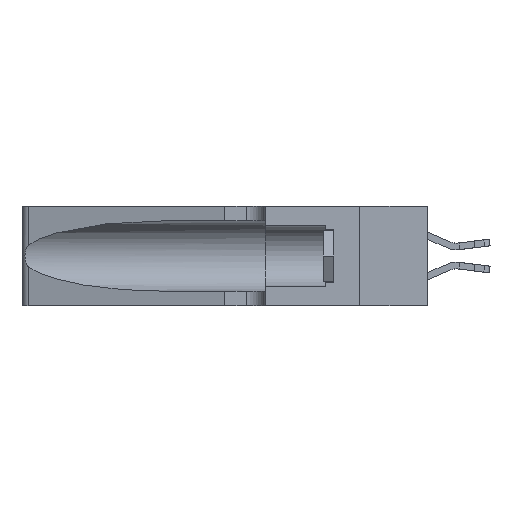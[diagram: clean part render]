
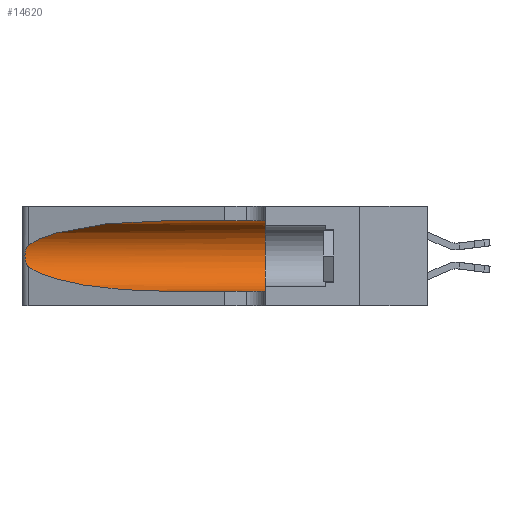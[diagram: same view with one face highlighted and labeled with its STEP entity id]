
A CAD part, left-side view. The second image highlights one B-rep face of the part: STEP entity #14620.
In plain terms, the highlighted cylindrical face has radius 3.308 mm (diameter 6.617 mm), a partial arc.
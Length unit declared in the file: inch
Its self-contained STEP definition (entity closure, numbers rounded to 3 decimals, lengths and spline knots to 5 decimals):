
#115 = LINE ( 'NONE', #6173, #20136 ) ;
#243 =( BOUNDED_CURVE ( )  B_SPLINE_CURVE ( 3, ( #4963, #20373, #3072, #16593 ),
 .UNSPECIFIED., .F., .F. ) 
 B_SPLINE_CURVE_WITH_KNOTS ( ( 4, 4 ),
 ( 3.44316, 4.71239 ),
 .UNSPECIFIED. ) 
 CURVE ( )  GEOMETRIC_REPRESENTATION_ITEM ( )  RATIONAL_B_SPLINE_CURVE ( ( 1., 0.87, 0.87, 1. ) ) 
 REPRESENTATION_ITEM ( '' )  );
#490 = ORIENTED_EDGE ( 'NONE', *, *, #7059, .T. ) ;
#665 = DIRECTION ( 'NONE',  ( 0., 0., -1. ) ) ;
#740 = VERTEX_POINT ( 'NONE', #21067 ) ;
#1482 = CARTESIAN_POINT ( 'NONE',  ( 0.25639, 1.23186, 0.15144 ) ) ;
#2315 =( BOUNDED_CURVE ( )  B_SPLINE_CURVE ( 3, ( #17032, #24825, #15292, #3704 ),
 .UNSPECIFIED., .F., .F. ) 
 B_SPLINE_CURVE_WITH_KNOTS ( ( 4, 4 ),
 ( 1.5708, 2.84003 ),
 .UNSPECIFIED. ) 
 CURVE ( )  GEOMETRIC_REPRESENTATION_ITEM ( )  RATIONAL_B_SPLINE_CURVE ( ( 1., 0.87, 0.87, 1. ) ) 
 REPRESENTATION_ITEM ( '' )  );
#3049 = EDGE_CURVE ( 'NONE', #3143, #14382, #3131, .T. ) ;
#3072 = CARTESIAN_POINT ( 'NONE',  ( 0.18966, 0.96281, 0.05475 ) ) ;
#3131 = B_SPLINE_CURVE_WITH_KNOTS ( 'NONE', 3,
 ( #5359, #8810, #10767, #18830, #7303, #20767, #9226, #22708, #11180, #24616, #13130, #1482, #15081, #3493 ),
 .UNSPECIFIED., .F., .F.,
 ( 4, 2, 2, 2, 2, 2, 4 ),
 ( 0., 0.00027, 0.00053, 0.00107, 0.0016, 0.00187, 0.00214 ),
 .UNSPECIFIED. ) ;
#3143 = VERTEX_POINT ( 'NONE', #21019 ) ;
#3493 = CARTESIAN_POINT ( 'NONE',  ( 0.25487, 1.22718, 0.14631 ) ) ;
#3704 = CARTESIAN_POINT ( 'NONE',  ( 0.25487, 1.22718, 0.22369 ) ) ;
#3903 = AXIS2_PLACEMENT_3D ( 'NONE', #9375, #22870, #11344 ) ;
#4679 = CARTESIAN_POINT ( 'NONE',  ( 0.1305, 0.35, 0.31525 ) ) ;
#4963 = CARTESIAN_POINT ( 'NONE',  ( 0.25487, 1.22718, 0.14631 ) ) ;
#5359 = CARTESIAN_POINT ( 'NONE',  ( 0.25487, 1.22718, 0.22369 ) ) ;
#5431 = ORIENTED_EDGE ( 'NONE', *, *, #17660, .F. ) ;
#5595 = FACE_OUTER_BOUND ( 'NONE', #14906, .T. ) ;
#5894 = CARTESIAN_POINT ( 'NONE',  ( 0.1305, 0.35, 0.05475 ) ) ;
#6173 = CARTESIAN_POINT ( 'NONE',  ( 0.1305, 1.61858, 0.31525 ) ) ;
#6381 = CARTESIAN_POINT ( 'NONE',  ( 0.1305, 1.61858, 0.05475 ) ) ;
#6445 = VERTEX_POINT ( 'NONE', #4679 ) ;
#7059 = EDGE_CURVE ( 'NONE', #740, #3143, #2315, .T. ) ;
#7303 = CARTESIAN_POINT ( 'NONE',  ( 0.25854, 1.2359, 0.20912 ) ) ;
#7697 = ORIENTED_EDGE ( 'NONE', *, *, #15644, .F. ) ;
#7951 = AXIS2_PLACEMENT_3D ( 'NONE', #12349, #18041, #665 ) ;
#8107 = DIRECTION ( 'NONE',  ( 0., -1., 0. ) ) ;
#8810 = CARTESIAN_POINT ( 'NONE',  ( 0.25555, 1.22994, 0.2215 ) ) ;
#9174 = ORIENTED_EDGE ( 'NONE', *, *, #11026, .T. ) ;
#9226 = CARTESIAN_POINT ( 'NONE',  ( 0.26075, 1.23896, 0.19203 ) ) ;
#9375 = CARTESIAN_POINT ( 'NONE',  ( 0.1305, 0.35, 0.185 ) ) ;
#9645 = VERTEX_POINT ( 'NONE', #5894 ) ;
#10767 = CARTESIAN_POINT ( 'NONE',  ( 0.25639, 1.23184, 0.21858 ) ) ;
#11026 = EDGE_CURVE ( 'NONE', #22867, #9645, #13200, .T. ) ;
#11180 = CARTESIAN_POINT ( 'NONE',  ( 0.26017, 1.23833, 0.17102 ) ) ;
#11344 = DIRECTION ( 'NONE',  ( 0., 0., 1. ) ) ;
#12025 = ORIENTED_EDGE ( 'NONE', *, *, #20662, .T. ) ;
#12349 = CARTESIAN_POINT ( 'NONE',  ( 0.1305, 1.61858, 0.185 ) ) ;
#13130 = CARTESIAN_POINT ( 'NONE',  ( 0.25789, 1.23486, 0.15765 ) ) ;
#13200 = LINE ( 'NONE', #6381, #22821 ) ;
#13603 = CARTESIAN_POINT ( 'NONE',  ( 0.25487, 1.22718, 0.14631 ) ) ;
#14382 = VERTEX_POINT ( 'NONE', #13603 ) ;
#14620 = ADVANCED_FACE ( 'NONE', ( #5595 ), #20366, .F. ) ;
#14906 = EDGE_LOOP ( 'NONE', ( #490, #15916, #12025, #9174, #7697, #5431 ) ) ;
#14977 = CIRCLE ( 'NONE', #3903, 0.13025 ) ;
#15081 = CARTESIAN_POINT ( 'NONE',  ( 0.25555, 1.22993, 0.14849 ) ) ;
#15292 = CARTESIAN_POINT ( 'NONE',  ( 0.2373, 1.15595, 0.28018 ) ) ;
#15644 = EDGE_CURVE ( 'NONE', #6445, #9645, #14977, .T. ) ;
#15916 = ORIENTED_EDGE ( 'NONE', *, *, #3049, .T. ) ;
#16593 = CARTESIAN_POINT ( 'NONE',  ( 0.1305, 0.72297, 0.05475 ) ) ;
#17032 = CARTESIAN_POINT ( 'NONE',  ( 0.1305, 0.72297, 0.31525 ) ) ;
#17660 = EDGE_CURVE ( 'NONE', #740, #6445, #115, .T. ) ;
#18041 = DIRECTION ( 'NONE',  ( 0., -1., 0. ) ) ;
#18830 = CARTESIAN_POINT ( 'NONE',  ( 0.25787, 1.23484, 0.2124 ) ) ;
#20136 = VECTOR ( 'NONE', #8107, 39.37008 ) ;
#20366 = CYLINDRICAL_SURFACE ( 'NONE', #7951, 0.13025 ) ;
#20373 = CARTESIAN_POINT ( 'NONE',  ( 0.2373, 1.15595, 0.08982 ) ) ;
#20662 = EDGE_CURVE ( 'NONE', #14382, #22867, #243, .T. ) ;
#20767 = CARTESIAN_POINT ( 'NONE',  ( 0.26018, 1.23835, 0.19895 ) ) ;
#21019 = CARTESIAN_POINT ( 'NONE',  ( 0.25487, 1.22718, 0.22369 ) ) ;
#21067 = CARTESIAN_POINT ( 'NONE',  ( 0.1305, 0.72297, 0.31525 ) ) ;
#21775 = DIRECTION ( 'NONE',  ( 0., -1., 0. ) ) ;
#22708 = CARTESIAN_POINT ( 'NONE',  ( 0.26075, 1.23896, 0.178 ) ) ;
#22821 = VECTOR ( 'NONE', #21775, 39.37008 ) ;
#22867 = VERTEX_POINT ( 'NONE', #23212 ) ;
#22870 = DIRECTION ( 'NONE',  ( 0., 1., 0. ) ) ;
#23212 = CARTESIAN_POINT ( 'NONE',  ( 0.1305, 0.72297, 0.05475 ) ) ;
#24616 = CARTESIAN_POINT ( 'NONE',  ( 0.25856, 1.23593, 0.16098 ) ) ;
#24825 = CARTESIAN_POINT ( 'NONE',  ( 0.18966, 0.96281, 0.31525 ) ) ;
